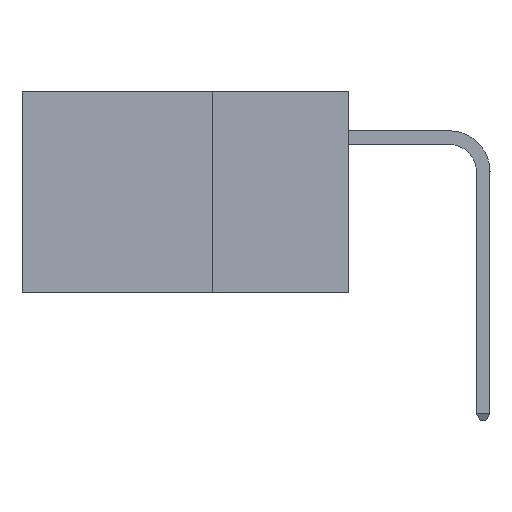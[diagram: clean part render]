
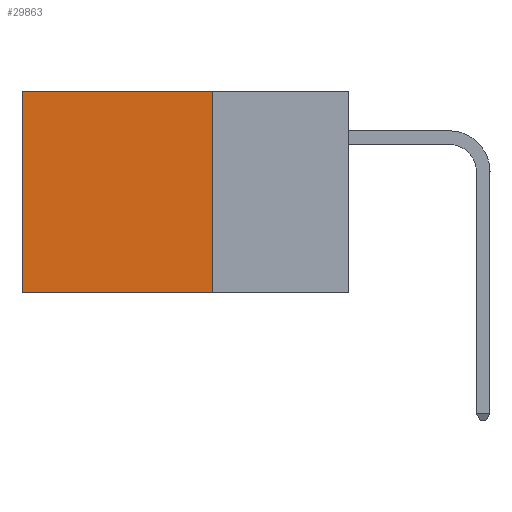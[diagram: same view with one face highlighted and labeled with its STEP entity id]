
A CAD part, left-side view. The second image highlights one B-rep face of the part: STEP entity #29863.
In plain terms, the highlighted planar face has unit normal (-1, 0, 0).
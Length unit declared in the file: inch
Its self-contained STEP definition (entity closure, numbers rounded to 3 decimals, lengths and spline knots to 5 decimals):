
#3515 = EDGE_CURVE ( 'NONE', #12378, #7056, #13716, .T. ) ;
#4091 = VECTOR ( 'NONE', #10449, 39.37008 ) ;
#4932 = EDGE_CURVE ( 'NONE', #12378, #9170, #30694, .T. ) ;
#4945 = CARTESIAN_POINT ( 'NONE',  ( 0.2875, 0.6, -0.37 ) ) ;
#7056 = VERTEX_POINT ( 'NONE', #16514 ) ;
#7702 = EDGE_CURVE ( 'NONE', #9170, #7710, #31399, .T. ) ;
#7710 = VERTEX_POINT ( 'NONE', #4945 ) ;
#8272 = DIRECTION ( 'NONE',  ( 1., 0., 0. ) ) ;
#9136 = VECTOR ( 'NONE', #22449, 39.37008 ) ;
#9170 = VERTEX_POINT ( 'NONE', #27594 ) ;
#9727 = CARTESIAN_POINT ( 'NONE',  ( 0.2875, 0.25, 0. ) ) ;
#10449 = DIRECTION ( 'NONE',  ( 0., 0., -1. ) ) ;
#12378 = VERTEX_POINT ( 'NONE', #9727 ) ;
#13459 = ORIENTED_EDGE ( 'NONE', *, *, #4932, .T. ) ;
#13716 = LINE ( 'NONE', #32420, #9136 ) ;
#13757 = VECTOR ( 'NONE', #21126, 39.37008 ) ;
#14328 = ORIENTED_EDGE ( 'NONE', *, *, #3515, .F. ) ;
#16514 = CARTESIAN_POINT ( 'NONE',  ( 0.2875, 0.25, -0.37 ) ) ;
#17654 = CARTESIAN_POINT ( 'NONE',  ( 0.2875, 0.25, 0. ) ) ;
#18008 = CARTESIAN_POINT ( 'NONE',  ( 0.2875, 0.6, 0. ) ) ;
#18374 = LINE ( 'NONE', #18546, #13757 ) ;
#18509 = VECTOR ( 'NONE', #26070, 39.37008 ) ;
#18546 = CARTESIAN_POINT ( 'NONE',  ( 0.2875, 0.25, -0.37 ) ) ;
#19086 = DIRECTION ( 'NONE',  ( 0., 0., -1. ) ) ;
#21126 = DIRECTION ( 'NONE',  ( 0., 1., 0. ) ) ;
#21298 = ORIENTED_EDGE ( 'NONE', *, *, #7702, .T. ) ;
#21322 = CARTESIAN_POINT ( 'NONE',  ( 0.2875, 0.25, 0. ) ) ;
#22449 = DIRECTION ( 'NONE',  ( 0., 0., -1. ) ) ;
#25440 = ORIENTED_EDGE ( 'NONE', *, *, #31818, .F. ) ;
#25771 = EDGE_LOOP ( 'NONE', ( #21298, #25440, #14328, #13459 ) ) ;
#26070 = DIRECTION ( 'NONE',  ( 0., 1., 0. ) ) ;
#26485 = FACE_OUTER_BOUND ( 'NONE', #25771, .T. ) ;
#27594 = CARTESIAN_POINT ( 'NONE',  ( 0.2875, 0.6, 0. ) ) ;
#29863 = ADVANCED_FACE ( 'NONE', ( #26485 ), #31968, .F. ) ;
#30112 = AXIS2_PLACEMENT_3D ( 'NONE', #21322, #8272, #19086 ) ;
#30694 = LINE ( 'NONE', #17654, #18509 ) ;
#31399 = LINE ( 'NONE', #18008, #4091 ) ;
#31818 = EDGE_CURVE ( 'NONE', #7056, #7710, #18374, .T. ) ;
#31968 = PLANE ( 'NONE',  #30112 ) ;
#32420 = CARTESIAN_POINT ( 'NONE',  ( 0.2875, 0.25, 0. ) ) ;
